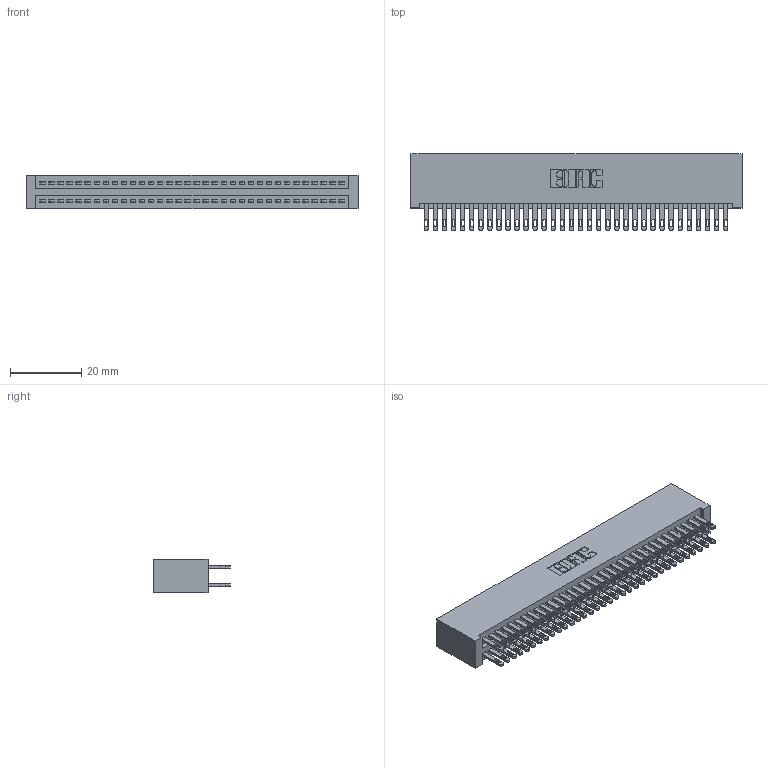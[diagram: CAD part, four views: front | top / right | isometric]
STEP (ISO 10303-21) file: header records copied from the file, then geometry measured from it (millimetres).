
FILE_DESCRIPTION (( 'STEP AP203' ), '1' );
FILE_NAME ('895-068-500-201.STEP', '2020-09-28T14:59:44', ( '' ), ( '' ), 'SwSTEP 2.0', 'SolidWorks 2020', '' );
FILE_SCHEMA (( 'CONFIG_CONTROL_DESIGN' ));
Length unit declared in the file: inch
Products named in the file (3): 845 Part_No Mounting Lugs; 345-292-001_345-293-100; 895-068-500-201
Assembly tree (69 placements, depth 2):
  895-068-500-201
    845 Part_No Mounting Lugs
    345-292-001_345-293-100  x68
Bounding box: 92.96 x 21.51 x 9.4 mm (x, y, z)
Volume: 9780.1 mm3; surface area: 15298.5 mm2
Topology: 69 solids, 69 shells, 3246 faces, 9905 edges, 6602 vertices
Faces by surface type: plane 1912, cylinder 1334
Entity records: 27407 total; most frequent: CARTESIAN_POINT 4600, ORIENTED_EDGE 4534, DIRECTION 4063, EDGE_CURVE 2267, VECTOR 2003, LINE 2003, VERTEX_POINT 1510, AXIS2_PLACEMENT_3D 1030
